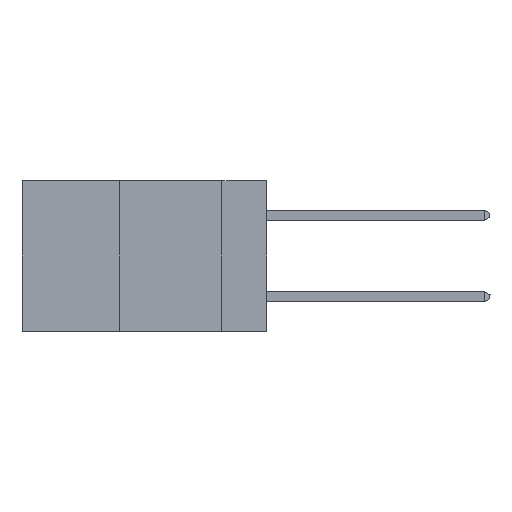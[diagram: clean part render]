
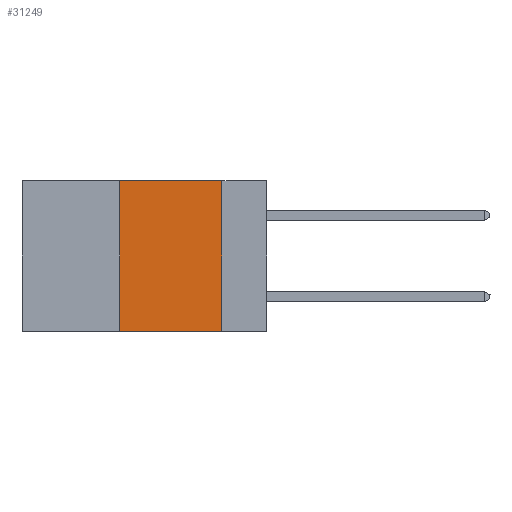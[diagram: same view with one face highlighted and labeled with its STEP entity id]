
A CAD part, left-side view. The second image highlights one B-rep face of the part: STEP entity #31249.
In plain terms, the highlighted planar face has unit normal (-1, 0, 0).
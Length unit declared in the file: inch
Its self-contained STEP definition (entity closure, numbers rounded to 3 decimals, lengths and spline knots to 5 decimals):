
#859 = LINE ( 'NONE', #21242, #35028 ) ;
#3183 = VECTOR ( 'NONE', #33389, 39.37008 ) ;
#4184 = CARTESIAN_POINT ( 'NONE',  ( 0., 0.11, 0. ) ) ;
#6020 = CARTESIAN_POINT ( 'NONE',  ( 0., 0.6, 0. ) ) ;
#8817 = EDGE_CURVE ( 'NONE', #16414, #35723, #39944, .T. ) ;
#8954 = ORIENTED_EDGE ( 'NONE', *, *, #11156, .F. ) ;
#9754 = ORIENTED_EDGE ( 'NONE', *, *, #8817, .F. ) ;
#11156 = EDGE_CURVE ( 'NONE', #27511, #16414, #41269, .T. ) ;
#12212 = DIRECTION ( 'NONE',  ( 0., 0., 1. ) ) ;
#12339 = CARTESIAN_POINT ( 'NONE',  ( 0., 0.11, 0. ) ) ;
#13693 = CARTESIAN_POINT ( 'NONE',  ( 0., 0.6, 0. ) ) ;
#16414 = VERTEX_POINT ( 'NONE', #36118 ) ;
#17761 = DIRECTION ( 'NONE',  ( 0., -1., 0. ) ) ;
#18531 = EDGE_LOOP ( 'NONE', ( #24988, #9754, #8954, #19169 ) ) ;
#19169 = ORIENTED_EDGE ( 'NONE', *, *, #41549, .T. ) ;
#19323 = DIRECTION ( 'NONE',  ( 0., 0., -1. ) ) ;
#21242 = CARTESIAN_POINT ( 'NONE',  ( 0., 0.6, -0.37 ) ) ;
#21607 = VECTOR ( 'NONE', #12212, 39.37008 ) ;
#24389 = AXIS2_PLACEMENT_3D ( 'NONE', #6020, #42768, #19323 ) ;
#24573 = VECTOR ( 'NONE', #29135, 39.37008 ) ;
#24601 = VERTEX_POINT ( 'NONE', #38606 ) ;
#24988 = ORIENTED_EDGE ( 'NONE', *, *, #29961, .F. ) ;
#27511 = VERTEX_POINT ( 'NONE', #28632 ) ;
#28632 = CARTESIAN_POINT ( 'NONE',  ( 0., 0.36, -0.37 ) ) ;
#29135 = DIRECTION ( 'NONE',  ( 0., 0., -1. ) ) ;
#29961 = EDGE_CURVE ( 'NONE', #35723, #24601, #33342, .T. ) ;
#31249 = ADVANCED_FACE ( 'NONE', ( #38433 ), #42194, .F. ) ;
#31617 = CARTESIAN_POINT ( 'NONE',  ( 0., 0.36, 0. ) ) ;
#33342 = LINE ( 'NONE', #12339, #24573 ) ;
#33389 = DIRECTION ( 'NONE',  ( 0., -1., 0. ) ) ;
#35028 = VECTOR ( 'NONE', #17761, 39.37008 ) ;
#35723 = VERTEX_POINT ( 'NONE', #4184 ) ;
#36118 = CARTESIAN_POINT ( 'NONE',  ( 0., 0.36, 0. ) ) ;
#38433 = FACE_OUTER_BOUND ( 'NONE', #18531, .T. ) ;
#38606 = CARTESIAN_POINT ( 'NONE',  ( 0., 0.11, -0.37 ) ) ;
#39944 = LINE ( 'NONE', #13693, #3183 ) ;
#41269 = LINE ( 'NONE', #31617, #21607 ) ;
#41549 = EDGE_CURVE ( 'NONE', #27511, #24601, #859, .T. ) ;
#42194 = PLANE ( 'NONE',  #24389 ) ;
#42768 = DIRECTION ( 'NONE',  ( 1., 0., 0. ) ) ;
